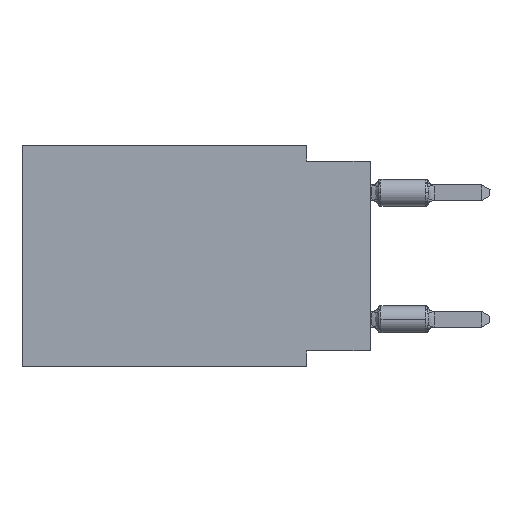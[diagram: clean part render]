
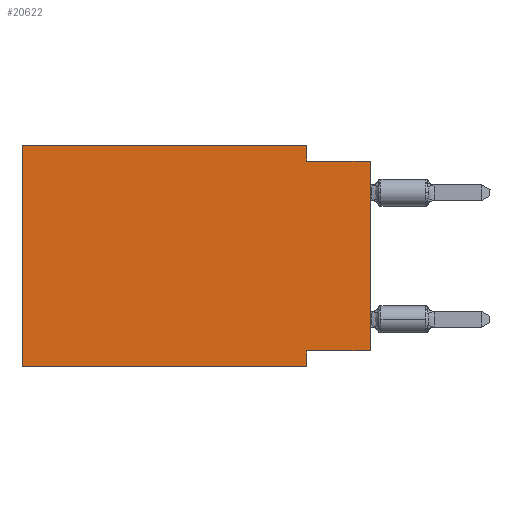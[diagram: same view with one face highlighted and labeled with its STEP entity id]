
A CAD part, left-side view. The second image highlights one B-rep face of the part: STEP entity #20622.
In plain terms, the highlighted planar face has unit normal (-1, 0, 0).
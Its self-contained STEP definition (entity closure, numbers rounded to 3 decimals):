
#19 = EDGE_CURVE ( 'NONE', #3398, #10048, #14993, .T. ) ;
#1278 = CARTESIAN_POINT ( 'NONE',  ( 0., 2.54, -8.255 ) ) ;
#2031 = CARTESIAN_POINT ( 'NONE',  ( 0., 13.97, 0. ) ) ;
#2337 = ORIENTED_EDGE ( 'NONE', *, *, #16832, .T. ) ;
#3043 = VERTEX_POINT ( 'NONE', #26128 ) ;
#3398 = VERTEX_POINT ( 'NONE', #15012 ) ;
#4033 = CARTESIAN_POINT ( 'NONE',  ( 0., 0., -0.635 ) ) ;
#4188 = ORIENTED_EDGE ( 'NONE', *, *, #14347, .F. ) ;
#4938 = LINE ( 'NONE', #26556, #11265 ) ;
#5316 = CARTESIAN_POINT ( 'NONE',  ( 0., 2.54, -0.635 ) ) ;
#5328 = ORIENTED_EDGE ( 'NONE', *, *, #7471, .T. ) ;
#5467 = CARTESIAN_POINT ( 'NONE',  ( 0., 0., -0.635 ) ) ;
#6018 = LINE ( 'NONE', #27793, #9834 ) ;
#6216 = PLANE ( 'NONE',  #22526 ) ;
#6597 = EDGE_CURVE ( 'NONE', #10048, #13645, #12211, .T. ) ;
#7076 = VERTEX_POINT ( 'NONE', #4033 ) ;
#7471 = EDGE_CURVE ( 'NONE', #3398, #3043, #20674, .T. ) ;
#7633 = CARTESIAN_POINT ( 'NONE',  ( 0., 2.54, 0. ) ) ;
#7918 = DIRECTION ( 'NONE',  ( 0., -1., 0. ) ) ;
#7937 = ORIENTED_EDGE ( 'NONE', *, *, #6597, .F. ) ;
#8767 = FACE_OUTER_BOUND ( 'NONE', #12757, .T. ) ;
#9057 = VERTEX_POINT ( 'NONE', #1278 ) ;
#9834 = VECTOR ( 'NONE', #23529, 1000. ) ;
#9863 = CARTESIAN_POINT ( 'NONE',  ( 0., 13.97, -8.89 ) ) ;
#9945 = CARTESIAN_POINT ( 'NONE',  ( 0., 2.54, 0. ) ) ;
#10048 = VERTEX_POINT ( 'NONE', #25905 ) ;
#11265 = VECTOR ( 'NONE', #18029, 1000. ) ;
#11520 = VERTEX_POINT ( 'NONE', #5316 ) ;
#11715 = VERTEX_POINT ( 'NONE', #21624 ) ;
#12018 = LINE ( 'NONE', #5467, #19013 ) ;
#12211 = LINE ( 'NONE', #20879, #25092 ) ;
#12757 = EDGE_LOOP ( 'NONE', ( #2337, #4188, #27806, #7937, #19786, #5328, #15969, #20598 ) ) ;
#12895 = LINE ( 'NONE', #24134, #25669 ) ;
#13645 = VERTEX_POINT ( 'NONE', #9945 ) ;
#13696 = VECTOR ( 'NONE', #14584, 1000. ) ;
#14155 = DIRECTION ( 'NONE',  ( 0., -1., 0. ) ) ;
#14347 = EDGE_CURVE ( 'NONE', #11520, #7076, #12018, .T. ) ;
#14476 = LINE ( 'NONE', #7633, #24752 ) ;
#14584 = DIRECTION ( 'NONE',  ( 0., 0., 1. ) ) ;
#14769 = DIRECTION ( 'NONE',  ( 1., 0., 0. ) ) ;
#14993 = LINE ( 'NONE', #2031, #13696 ) ;
#15012 = CARTESIAN_POINT ( 'NONE',  ( 0., 13.97, -8.89 ) ) ;
#15046 = DIRECTION ( 'NONE',  ( 0., 0., -1. ) ) ;
#15315 = DIRECTION ( 'NONE',  ( 0., 1., 0. ) ) ;
#15969 = ORIENTED_EDGE ( 'NONE', *, *, #25615, .F. ) ;
#16832 = EDGE_CURVE ( 'NONE', #11715, #7076, #4938, .T. ) ;
#17731 = VECTOR ( 'NONE', #18819, 1000. ) ;
#18029 = DIRECTION ( 'NONE',  ( 0., 0., 1. ) ) ;
#18254 = EDGE_CURVE ( 'NONE', #11715, #9057, #12895, .T. ) ;
#18819 = DIRECTION ( 'NONE',  ( 0., -1., 0. ) ) ;
#19013 = VECTOR ( 'NONE', #14155, 1000. ) ;
#19786 = ORIENTED_EDGE ( 'NONE', *, *, #19, .F. ) ;
#20598 = ORIENTED_EDGE ( 'NONE', *, *, #18254, .F. ) ;
#20622 = ADVANCED_FACE ( 'NONE', ( #8767 ), #6216, .F. ) ;
#20674 = LINE ( 'NONE', #9863, #17731 ) ;
#20879 = CARTESIAN_POINT ( 'NONE',  ( 0., 13.97, 0. ) ) ;
#21624 = CARTESIAN_POINT ( 'NONE',  ( 0., 0., -8.255 ) ) ;
#21732 = CARTESIAN_POINT ( 'NONE',  ( 0., 13.97, 0. ) ) ;
#22526 = AXIS2_PLACEMENT_3D ( 'NONE', #21732, #14769, #15046 ) ;
#22722 = DIRECTION ( 'NONE',  ( 0., 0., -1. ) ) ;
#23311 = EDGE_CURVE ( 'NONE', #13645, #11520, #14476, .T. ) ;
#23529 = DIRECTION ( 'NONE',  ( 0., 0., -1. ) ) ;
#24134 = CARTESIAN_POINT ( 'NONE',  ( 0., 0., -8.255 ) ) ;
#24752 = VECTOR ( 'NONE', #22722, 1000. ) ;
#25092 = VECTOR ( 'NONE', #7918, 1000. ) ;
#25615 = EDGE_CURVE ( 'NONE', #9057, #3043, #6018, .T. ) ;
#25669 = VECTOR ( 'NONE', #15315, 1000. ) ;
#25905 = CARTESIAN_POINT ( 'NONE',  ( 0., 13.97, 0. ) ) ;
#26128 = CARTESIAN_POINT ( 'NONE',  ( 0., 2.54, -8.89 ) ) ;
#26556 = CARTESIAN_POINT ( 'NONE',  ( 0., 0., 0. ) ) ;
#27793 = CARTESIAN_POINT ( 'NONE',  ( 0., 2.54, -8.89 ) ) ;
#27806 = ORIENTED_EDGE ( 'NONE', *, *, #23311, .F. ) ;
